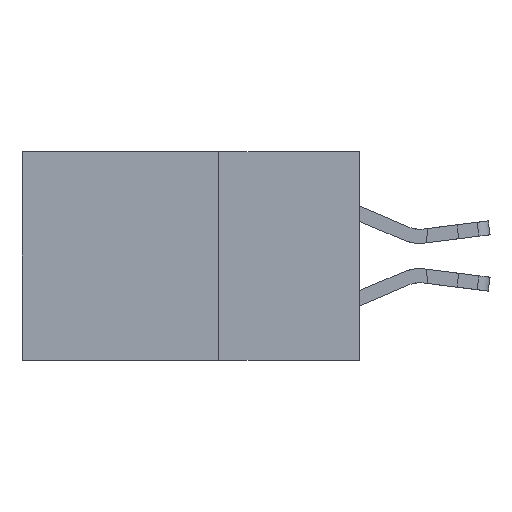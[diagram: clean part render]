
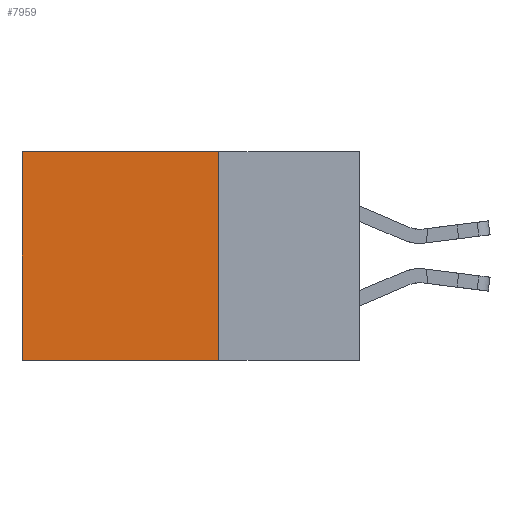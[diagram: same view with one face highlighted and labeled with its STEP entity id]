
A CAD part, left-side view. The second image highlights one B-rep face of the part: STEP entity #7959.
In plain terms, the highlighted planar face has unit normal (-1, 0, 0).
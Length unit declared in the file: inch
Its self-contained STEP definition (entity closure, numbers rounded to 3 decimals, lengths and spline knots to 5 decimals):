
#986 = CARTESIAN_POINT ( 'NONE',  ( 0.2875, 0.25, 0. ) ) ;
#1327 = DIRECTION ( 'NONE',  ( 0., 0., -1. ) ) ;
#1482 = LINE ( 'NONE', #23572, #22232 ) ;
#2371 = DIRECTION ( 'NONE',  ( 1., 0., 0. ) ) ;
#2938 = EDGE_CURVE ( 'NONE', #17130, #3386, #8423, .T. ) ;
#3386 = VERTEX_POINT ( 'NONE', #22551 ) ;
#4353 = CARTESIAN_POINT ( 'NONE',  ( 0.2875, 0.6, 0. ) ) ;
#4651 = CARTESIAN_POINT ( 'NONE',  ( 0.2875, 0.25, -0.37 ) ) ;
#5127 = FACE_OUTER_BOUND ( 'NONE', #19678, .T. ) ;
#5331 = CARTESIAN_POINT ( 'NONE',  ( 0.2875, 0.6, 0. ) ) ;
#5460 = VECTOR ( 'NONE', #1327, 39.37008 ) ;
#6135 = VERTEX_POINT ( 'NONE', #4353 ) ;
#7317 = VECTOR ( 'NONE', #19725, 39.37008 ) ;
#7959 = ADVANCED_FACE ( 'NONE', ( #5127 ), #10998, .F. ) ;
#8423 = LINE ( 'NONE', #20023, #13437 ) ;
#9358 = DIRECTION ( 'NONE',  ( 0., 0., -1. ) ) ;
#9895 = LINE ( 'NONE', #5331, #5460 ) ;
#10998 = PLANE ( 'NONE',  #20535 ) ;
#11635 = ORIENTED_EDGE ( 'NONE', *, *, #18734, .F. ) ;
#12611 = LINE ( 'NONE', #23710, #7317 ) ;
#13437 = VECTOR ( 'NONE', #22065, 39.37008 ) ;
#15242 = DIRECTION ( 'NONE',  ( 0., 0., -1. ) ) ;
#16221 = VERTEX_POINT ( 'NONE', #22279 ) ;
#17130 = VERTEX_POINT ( 'NONE', #4651 ) ;
#18734 = EDGE_CURVE ( 'NONE', #16221, #17130, #1482, .T. ) ;
#19678 = EDGE_LOOP ( 'NONE', ( #19771, #25379, #11635, #21849 ) ) ;
#19725 = DIRECTION ( 'NONE',  ( 0., 1., 0. ) ) ;
#19771 = ORIENTED_EDGE ( 'NONE', *, *, #20037, .T. ) ;
#20023 = CARTESIAN_POINT ( 'NONE',  ( 0.2875, 0.25, -0.37 ) ) ;
#20037 = EDGE_CURVE ( 'NONE', #6135, #3386, #9895, .T. ) ;
#20535 = AXIS2_PLACEMENT_3D ( 'NONE', #986, #2371, #9358 ) ;
#21849 = ORIENTED_EDGE ( 'NONE', *, *, #21859, .T. ) ;
#21859 = EDGE_CURVE ( 'NONE', #16221, #6135, #12611, .T. ) ;
#22065 = DIRECTION ( 'NONE',  ( 0., 1., 0. ) ) ;
#22232 = VECTOR ( 'NONE', #15242, 39.37008 ) ;
#22279 = CARTESIAN_POINT ( 'NONE',  ( 0.2875, 0.25, 0. ) ) ;
#22551 = CARTESIAN_POINT ( 'NONE',  ( 0.2875, 0.6, -0.37 ) ) ;
#23572 = CARTESIAN_POINT ( 'NONE',  ( 0.2875, 0.25, 0. ) ) ;
#23710 = CARTESIAN_POINT ( 'NONE',  ( 0.2875, 0.25, 0. ) ) ;
#25379 = ORIENTED_EDGE ( 'NONE', *, *, #2938, .F. ) ;
